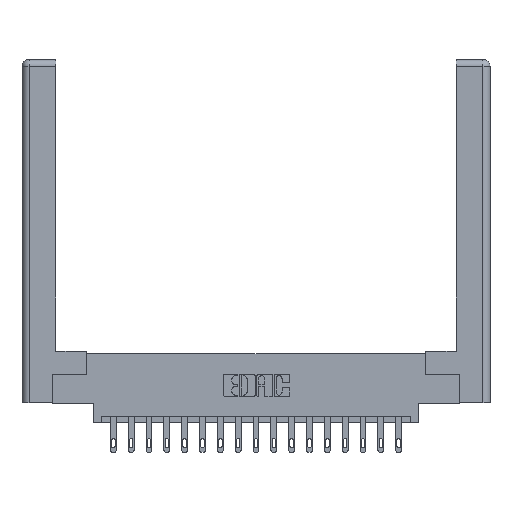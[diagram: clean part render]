
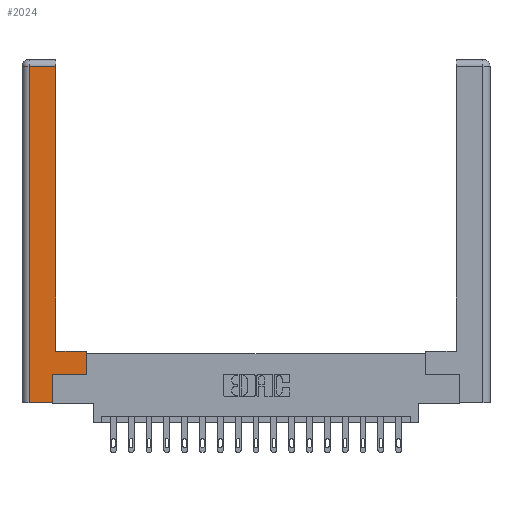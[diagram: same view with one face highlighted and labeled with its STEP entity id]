
A CAD part, top view. The second image highlights one B-rep face of the part: STEP entity #2024.
In plain terms, the highlighted planar face has unit normal (0, 0, 1).
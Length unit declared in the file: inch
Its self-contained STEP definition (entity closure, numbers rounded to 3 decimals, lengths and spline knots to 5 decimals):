
#140 = CARTESIAN_POINT ( 'NONE',  ( 0.0615, 2.94, 0. ) ) ;
#314 = CARTESIAN_POINT ( 'NONE',  ( 0.565, 0.45, 0. ) ) ;
#555 = VECTOR ( 'NONE', #3978, 39.37008 ) ;
#954 = LINE ( 'NONE', #8705, #3326 ) ;
#1042 = EDGE_CURVE ( 'NONE', #2907, #17936, #954, .T. ) ;
#1254 = LINE ( 'NONE', #18853, #8725 ) ;
#1376 = DIRECTION ( 'NONE',  ( -1., 0., 0. ) ) ;
#2024 = ADVANCED_FACE ( 'NONE', ( #7731 ), #4645, .F. ) ;
#2619 = CARTESIAN_POINT ( 'NONE',  ( 0.265, 0.245, 0. ) ) ;
#2826 = EDGE_CURVE ( 'NONE', #14369, #14513, #5117, .T. ) ;
#2860 = VERTEX_POINT ( 'NONE', #15886 ) ;
#2907 = VERTEX_POINT ( 'NONE', #18820 ) ;
#3326 = VECTOR ( 'NONE', #16211, 39.37008 ) ;
#3712 = EDGE_CURVE ( 'NONE', #17936, #2860, #11106, .T. ) ;
#3978 = DIRECTION ( 'NONE',  ( 0., -1., 0. ) ) ;
#4313 = EDGE_LOOP ( 'NONE', ( #16146, #13784, #15831, #8831, #18243, #6604, #17346, #5108 ) ) ;
#4359 = CARTESIAN_POINT ( 'NONE',  ( 0.265, 0., 0. ) ) ;
#4493 = DIRECTION ( 'NONE',  ( 0., 0., -1. ) ) ;
#4645 = PLANE ( 'NONE',  #7080 ) ;
#5100 = LINE ( 'NONE', #6936, #5776 ) ;
#5108 = ORIENTED_EDGE ( 'NONE', *, *, #5813, .T. ) ;
#5111 = CARTESIAN_POINT ( 'NONE',  ( 0.0615, 0., 0. ) ) ;
#5117 = LINE ( 'NONE', #5305, #16429 ) ;
#5305 = CARTESIAN_POINT ( 'NONE',  ( 0.565, 0.245, 0. ) ) ;
#5744 = EDGE_CURVE ( 'NONE', #2860, #10753, #8951, .T. ) ;
#5776 = VECTOR ( 'NONE', #12976, 39.37008 ) ;
#5813 = EDGE_CURVE ( 'NONE', #16027, #2907, #1254, .T. ) ;
#6576 = EDGE_CURVE ( 'NONE', #19002, #14369, #5100, .T. ) ;
#6604 = ORIENTED_EDGE ( 'NONE', *, *, #2826, .T. ) ;
#6936 = CARTESIAN_POINT ( 'NONE',  ( 0.265, 0.245, 0. ) ) ;
#7080 = AXIS2_PLACEMENT_3D ( 'NONE', #14958, #4493, #1376 ) ;
#7731 = FACE_OUTER_BOUND ( 'NONE', #4313, .T. ) ;
#8705 = CARTESIAN_POINT ( 'NONE',  ( 0.295, 3., 0. ) ) ;
#8725 = VECTOR ( 'NONE', #10100, 39.37008 ) ;
#8831 = ORIENTED_EDGE ( 'NONE', *, *, #13924, .T. ) ;
#8951 = LINE ( 'NONE', #5111, #555 ) ;
#9143 = DIRECTION ( 'NONE',  ( -1., 0., 0. ) ) ;
#9272 = CARTESIAN_POINT ( 'NONE',  ( 0.565, 0.45, 0. ) ) ;
#9525 = DIRECTION ( 'NONE',  ( 1., 0., 0. ) ) ;
#10100 = DIRECTION ( 'NONE',  ( -1., 0., 0. ) ) ;
#10426 = VECTOR ( 'NONE', #9143, 39.37008 ) ;
#10753 = VERTEX_POINT ( 'NONE', #14581 ) ;
#10921 = DIRECTION ( 'NONE',  ( 1., 0., 0. ) ) ;
#11106 = LINE ( 'NONE', #140, #10426 ) ;
#11472 = VECTOR ( 'NONE', #10921, 39.37008 ) ;
#11695 = LINE ( 'NONE', #18311, #11472 ) ;
#11888 = DIRECTION ( 'NONE',  ( 0., 1., 0. ) ) ;
#12058 = CARTESIAN_POINT ( 'NONE',  ( 0.565, 0.245, 0. ) ) ;
#12976 = DIRECTION ( 'NONE',  ( 0., 1., 0. ) ) ;
#13435 = LINE ( 'NONE', #314, #15993 ) ;
#13784 = ORIENTED_EDGE ( 'NONE', *, *, #3712, .T. ) ;
#13924 = EDGE_CURVE ( 'NONE', #10753, #19002, #11695, .T. ) ;
#14369 = VERTEX_POINT ( 'NONE', #2619 ) ;
#14513 = VERTEX_POINT ( 'NONE', #12058 ) ;
#14581 = CARTESIAN_POINT ( 'NONE',  ( 0.0615, 0., 0. ) ) ;
#14958 = CARTESIAN_POINT ( 'NONE',  ( 0., 0., 0. ) ) ;
#15460 = EDGE_CURVE ( 'NONE', #14513, #16027, #13435, .T. ) ;
#15831 = ORIENTED_EDGE ( 'NONE', *, *, #5744, .T. ) ;
#15886 = CARTESIAN_POINT ( 'NONE',  ( 0.0615, 2.94, 0. ) ) ;
#15993 = VECTOR ( 'NONE', #11888, 39.37008 ) ;
#16027 = VERTEX_POINT ( 'NONE', #9272 ) ;
#16146 = ORIENTED_EDGE ( 'NONE', *, *, #1042, .T. ) ;
#16211 = DIRECTION ( 'NONE',  ( 0., 1., 0. ) ) ;
#16429 = VECTOR ( 'NONE', #9525, 39.37008 ) ;
#17346 = ORIENTED_EDGE ( 'NONE', *, *, #15460, .T. ) ;
#17890 = CARTESIAN_POINT ( 'NONE',  ( 0.295, 2.94, 0. ) ) ;
#17936 = VERTEX_POINT ( 'NONE', #17890 ) ;
#18243 = ORIENTED_EDGE ( 'NONE', *, *, #6576, .T. ) ;
#18311 = CARTESIAN_POINT ( 'NONE',  ( 0.265, 0., 0. ) ) ;
#18820 = CARTESIAN_POINT ( 'NONE',  ( 0.295, 0.45, 0. ) ) ;
#18853 = CARTESIAN_POINT ( 'NONE',  ( 0.295, 0.45, 0. ) ) ;
#19002 = VERTEX_POINT ( 'NONE', #4359 ) ;
